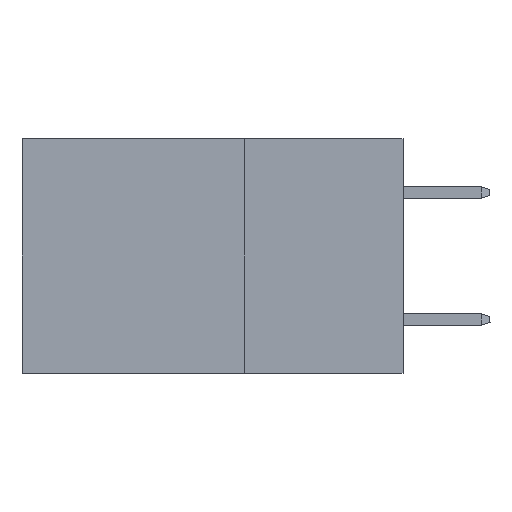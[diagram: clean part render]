
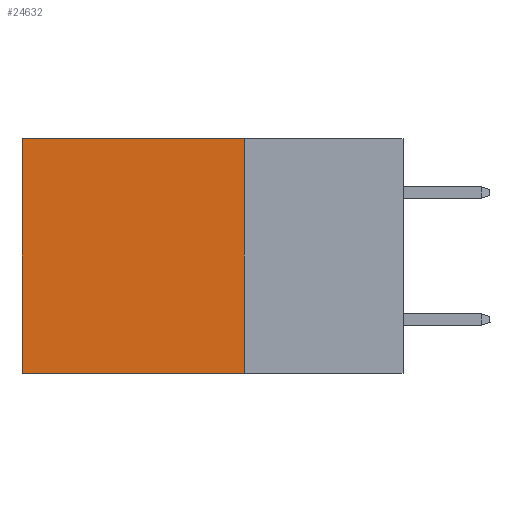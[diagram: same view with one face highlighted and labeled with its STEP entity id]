
A CAD part, left-side view. The second image highlights one B-rep face of the part: STEP entity #24632.
In plain terms, the highlighted planar face has unit normal (-1, 0, 0).
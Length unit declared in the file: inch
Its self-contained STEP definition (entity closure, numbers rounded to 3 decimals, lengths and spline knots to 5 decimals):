
#855 = DIRECTION ( 'NONE',  ( 0., 1., 0. ) ) ;
#1361 = ORIENTED_EDGE ( 'NONE', *, *, #13134, .F. ) ;
#1614 = EDGE_LOOP ( 'NONE', ( #14820, #1361, #3407, #13153 ) ) ;
#2308 = LINE ( 'NONE', #4774, #14197 ) ;
#2491 = CARTESIAN_POINT ( 'NONE',  ( 0.2875, 0.6, -0.37 ) ) ;
#3129 = PLANE ( 'NONE',  #12548 ) ;
#3407 = ORIENTED_EDGE ( 'NONE', *, *, #23437, .F. ) ;
#4774 = CARTESIAN_POINT ( 'NONE',  ( 0.2875, 0.6, 0. ) ) ;
#4910 = LINE ( 'NONE', #13177, #22547 ) ;
#5731 = CARTESIAN_POINT ( 'NONE',  ( 0.2875, 0.25, 0. ) ) ;
#6116 = CARTESIAN_POINT ( 'NONE',  ( 0.2875, 0.25, -0.37 ) ) ;
#6726 = VERTEX_POINT ( 'NONE', #6116 ) ;
#6802 = FACE_OUTER_BOUND ( 'NONE', #1614, .T. ) ;
#7910 = VERTEX_POINT ( 'NONE', #20820 ) ;
#8896 = LINE ( 'NONE', #5731, #14180 ) ;
#9289 = DIRECTION ( 'NONE',  ( 0., 0., -1. ) ) ;
#11071 = EDGE_CURVE ( 'NONE', #7910, #18704, #2308, .T. ) ;
#12548 = AXIS2_PLACEMENT_3D ( 'NONE', #23325, #14929, #9289 ) ;
#12940 = VECTOR ( 'NONE', #855, 39.37008 ) ;
#13134 = EDGE_CURVE ( 'NONE', #6726, #18704, #4910, .T. ) ;
#13153 = ORIENTED_EDGE ( 'NONE', *, *, #24254, .T. ) ;
#13177 = CARTESIAN_POINT ( 'NONE',  ( 0.2875, 0.25, -0.37 ) ) ;
#14180 = VECTOR ( 'NONE', #17409, 39.37008 ) ;
#14197 = VECTOR ( 'NONE', #24728, 39.37008 ) ;
#14760 = DIRECTION ( 'NONE',  ( 0., 1., 0. ) ) ;
#14820 = ORIENTED_EDGE ( 'NONE', *, *, #11071, .T. ) ;
#14929 = DIRECTION ( 'NONE',  ( 1., 0., 0. ) ) ;
#17409 = DIRECTION ( 'NONE',  ( 0., 0., -1. ) ) ;
#18704 = VERTEX_POINT ( 'NONE', #2491 ) ;
#20820 = CARTESIAN_POINT ( 'NONE',  ( 0.2875, 0.6, 0. ) ) ;
#20905 = CARTESIAN_POINT ( 'NONE',  ( 0.2875, 0.25, 0. ) ) ;
#22547 = VECTOR ( 'NONE', #14760, 39.37008 ) ;
#23325 = CARTESIAN_POINT ( 'NONE',  ( 0.2875, 0.25, 0. ) ) ;
#23437 = EDGE_CURVE ( 'NONE', #25717, #6726, #8896, .T. ) ;
#24016 = CARTESIAN_POINT ( 'NONE',  ( 0.2875, 0.25, 0. ) ) ;
#24254 = EDGE_CURVE ( 'NONE', #25717, #7910, #24462, .T. ) ;
#24462 = LINE ( 'NONE', #20905, #12940 ) ;
#24632 = ADVANCED_FACE ( 'NONE', ( #6802 ), #3129, .F. ) ;
#24728 = DIRECTION ( 'NONE',  ( 0., 0., -1. ) ) ;
#25717 = VERTEX_POINT ( 'NONE', #24016 ) ;
